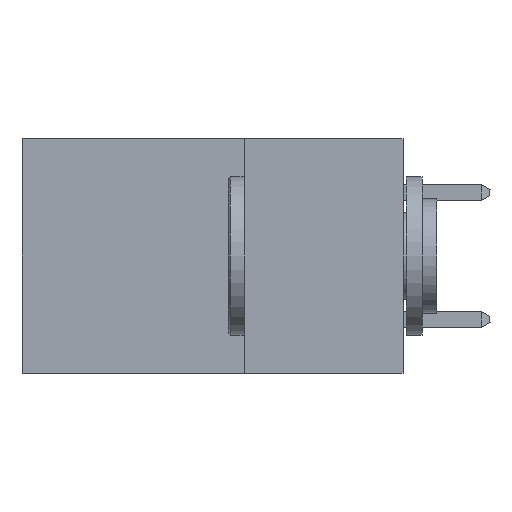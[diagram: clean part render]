
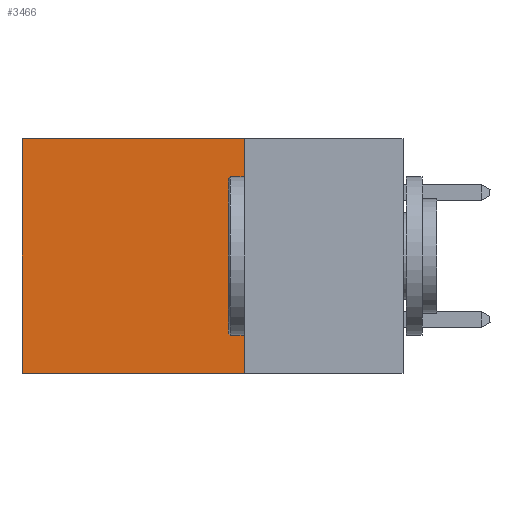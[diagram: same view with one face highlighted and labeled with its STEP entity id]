
A CAD part, left-side view. The second image highlights one B-rep face of the part: STEP entity #3466.
In plain terms, the highlighted planar face has unit normal (-1, 0, 0).
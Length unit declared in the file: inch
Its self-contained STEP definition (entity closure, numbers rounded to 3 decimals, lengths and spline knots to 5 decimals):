
#4 = VERTEX_POINT ( 'NONE', #11348 ) ;
#455 = EDGE_LOOP ( 'NONE', ( #25307, #8484, #32662, #16351 ) ) ;
#2146 = DIRECTION ( 'NONE',  ( 0., 0., -1. ) ) ;
#3466 = ADVANCED_FACE ( 'NONE', ( #19063 ), #26352, .F. ) ;
#6473 = CARTESIAN_POINT ( 'NONE',  ( 0.2875, 0.25, -0.37 ) ) ;
#6607 = EDGE_CURVE ( 'NONE', #4, #16187, #7954, .T. ) ;
#6678 = EDGE_CURVE ( 'NONE', #24688, #4, #26002, .T. ) ;
#7017 = EDGE_CURVE ( 'NONE', #24688, #22445, #8766, .T. ) ;
#7954 = LINE ( 'NONE', #24640, #27688 ) ;
#8484 = ORIENTED_EDGE ( 'NONE', *, *, #21165, .F. ) ;
#8766 = LINE ( 'NONE', #15580, #29349 ) ;
#8949 = DIRECTION ( 'NONE',  ( 0., 1., 0. ) ) ;
#9125 = CARTESIAN_POINT ( 'NONE',  ( 0.2875, 0.25, 0. ) ) ;
#10301 = CARTESIAN_POINT ( 'NONE',  ( 0.2875, 0.25, 0. ) ) ;
#11348 = CARTESIAN_POINT ( 'NONE',  ( 0.2875, 0.6, 0. ) ) ;
#12952 = DIRECTION ( 'NONE',  ( 1., 0., 0. ) ) ;
#15580 = CARTESIAN_POINT ( 'NONE',  ( 0.2875, 0.25, 0. ) ) ;
#16187 = VERTEX_POINT ( 'NONE', #26263 ) ;
#16351 = ORIENTED_EDGE ( 'NONE', *, *, #6678, .T. ) ;
#17228 = DIRECTION ( 'NONE',  ( 0., 1., 0. ) ) ;
#17541 = CARTESIAN_POINT ( 'NONE',  ( 0.2875, 0.25, -0.37 ) ) ;
#19063 = FACE_OUTER_BOUND ( 'NONE', #455, .T. ) ;
#19648 = VECTOR ( 'NONE', #8949, 39.37008 ) ;
#21165 = EDGE_CURVE ( 'NONE', #22445, #16187, #31380, .T. ) ;
#22027 = DIRECTION ( 'NONE',  ( 0., 0., -1. ) ) ;
#22445 = VERTEX_POINT ( 'NONE', #17541 ) ;
#23338 = VECTOR ( 'NONE', #17228, 39.37008 ) ;
#24640 = CARTESIAN_POINT ( 'NONE',  ( 0.2875, 0.6, 0. ) ) ;
#24688 = VERTEX_POINT ( 'NONE', #9125 ) ;
#24985 = CARTESIAN_POINT ( 'NONE',  ( 0.2875, 0.25, 0. ) ) ;
#25246 = AXIS2_PLACEMENT_3D ( 'NONE', #10301, #12952, #31789 ) ;
#25307 = ORIENTED_EDGE ( 'NONE', *, *, #6607, .T. ) ;
#26002 = LINE ( 'NONE', #24985, #19648 ) ;
#26263 = CARTESIAN_POINT ( 'NONE',  ( 0.2875, 0.6, -0.37 ) ) ;
#26352 = PLANE ( 'NONE',  #25246 ) ;
#27688 = VECTOR ( 'NONE', #22027, 39.37008 ) ;
#29349 = VECTOR ( 'NONE', #2146, 39.37008 ) ;
#31380 = LINE ( 'NONE', #6473, #23338 ) ;
#31789 = DIRECTION ( 'NONE',  ( 0., 0., -1. ) ) ;
#32662 = ORIENTED_EDGE ( 'NONE', *, *, #7017, .F. ) ;
